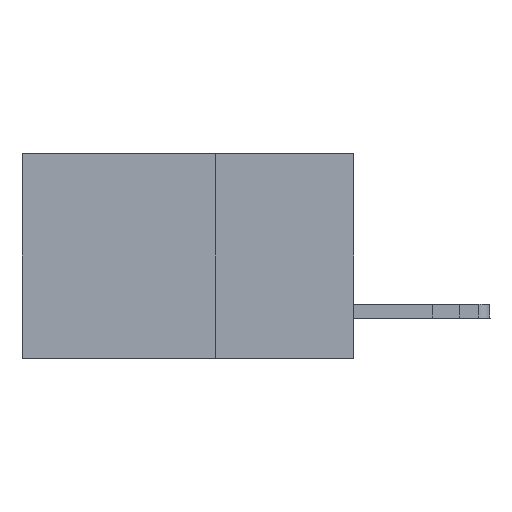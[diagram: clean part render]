
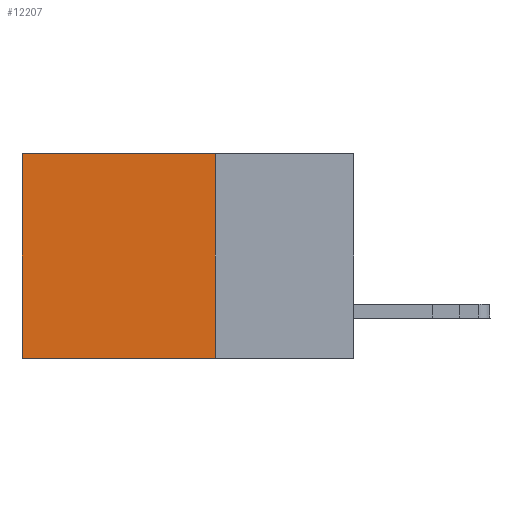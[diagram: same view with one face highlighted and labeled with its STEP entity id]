
A CAD part, left-side view. The second image highlights one B-rep face of the part: STEP entity #12207.
In plain terms, the highlighted planar face has unit normal (-1, 0, 0).
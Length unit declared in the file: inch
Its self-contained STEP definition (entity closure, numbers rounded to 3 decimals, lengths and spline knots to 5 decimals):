
#1130 = ORIENTED_EDGE ( 'NONE', *, *, #15975, .T. ) ;
#1554 = CARTESIAN_POINT ( 'NONE',  ( 0.2875, 0.25, 0. ) ) ;
#1636 = VERTEX_POINT ( 'NONE', #5452 ) ;
#2338 = LINE ( 'NONE', #14353, #6362 ) ;
#2929 = CARTESIAN_POINT ( 'NONE',  ( 0.2875, 0.25, 0. ) ) ;
#4022 = DIRECTION ( 'NONE',  ( 0., 0., -1. ) ) ;
#4660 = DIRECTION ( 'NONE',  ( 0., 1., 0. ) ) ;
#5003 = CARTESIAN_POINT ( 'NONE',  ( 0.2875, 0.25, -0.37 ) ) ;
#5206 = ORIENTED_EDGE ( 'NONE', *, *, #16671, .T. ) ;
#5452 = CARTESIAN_POINT ( 'NONE',  ( 0.2875, 0.6, 0. ) ) ;
#6036 = DIRECTION ( 'NONE',  ( 0., 1., 0. ) ) ;
#6362 = VECTOR ( 'NONE', #6036, 39.37008 ) ;
#7675 = PLANE ( 'NONE',  #7966 ) ;
#7966 = AXIS2_PLACEMENT_3D ( 'NONE', #17601, #9369, #20805 ) ;
#8575 = CARTESIAN_POINT ( 'NONE',  ( 0.2875, 0.25, 0. ) ) ;
#8648 = LINE ( 'NONE', #14076, #13049 ) ;
#8955 = VECTOR ( 'NONE', #11874, 39.37008 ) ;
#9367 = EDGE_LOOP ( 'NONE', ( #5206, #17998, #14979, #1130 ) ) ;
#9369 = DIRECTION ( 'NONE',  ( 1., 0., 0. ) ) ;
#9456 = LINE ( 'NONE', #2929, #19202 ) ;
#9645 = VERTEX_POINT ( 'NONE', #5003 ) ;
#10508 = LINE ( 'NONE', #8575, #8955 ) ;
#11874 = DIRECTION ( 'NONE',  ( 0., 0., -1. ) ) ;
#12207 = ADVANCED_FACE ( 'NONE', ( #18395 ), #7675, .F. ) ;
#12444 = VERTEX_POINT ( 'NONE', #13258 ) ;
#13049 = VECTOR ( 'NONE', #4022, 39.37008 ) ;
#13258 = CARTESIAN_POINT ( 'NONE',  ( 0.2875, 0.6, -0.37 ) ) ;
#14076 = CARTESIAN_POINT ( 'NONE',  ( 0.2875, 0.6, 0. ) ) ;
#14353 = CARTESIAN_POINT ( 'NONE',  ( 0.2875, 0.25, -0.37 ) ) ;
#14979 = ORIENTED_EDGE ( 'NONE', *, *, #15496, .F. ) ;
#15168 = EDGE_CURVE ( 'NONE', #9645, #12444, #2338, .T. ) ;
#15496 = EDGE_CURVE ( 'NONE', #16097, #9645, #10508, .T. ) ;
#15975 = EDGE_CURVE ( 'NONE', #16097, #1636, #9456, .T. ) ;
#16097 = VERTEX_POINT ( 'NONE', #1554 ) ;
#16671 = EDGE_CURVE ( 'NONE', #1636, #12444, #8648, .T. ) ;
#17601 = CARTESIAN_POINT ( 'NONE',  ( 0.2875, 0.25, 0. ) ) ;
#17998 = ORIENTED_EDGE ( 'NONE', *, *, #15168, .F. ) ;
#18395 = FACE_OUTER_BOUND ( 'NONE', #9367, .T. ) ;
#19202 = VECTOR ( 'NONE', #4660, 39.37008 ) ;
#20805 = DIRECTION ( 'NONE',  ( 0., 0., -1. ) ) ;
